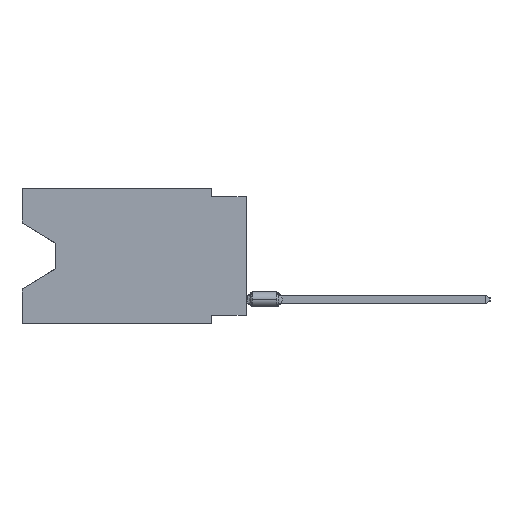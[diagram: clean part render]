
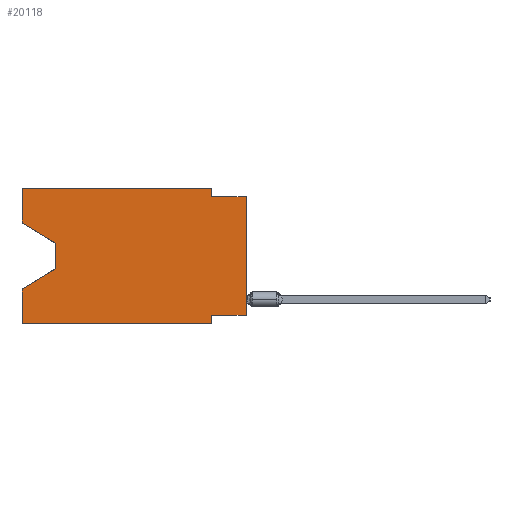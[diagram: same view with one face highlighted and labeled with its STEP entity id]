
A CAD part, left-side view. The second image highlights one B-rep face of the part: STEP entity #20118.
In plain terms, the highlighted planar face has unit normal (-1, 0, 0).
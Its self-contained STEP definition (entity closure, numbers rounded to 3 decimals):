
#1104 = VECTOR ( 'NONE', #51613, 1000. ) ;
#1359 = ORIENTED_EDGE ( 'NONE', *, *, #42672, .T. ) ;
#1464 = EDGE_CURVE ( 'NONE', #30477, #52670, #32960, .T. ) ;
#1602 = CARTESIAN_POINT ( 'NONE',  ( 0., 13.97, -5.893 ) ) ;
#2271 = EDGE_LOOP ( 'NONE', ( #1359, #35924, #19201, #23633, #43692, #17999, #37545, #6547, #33338, #36070, #18843, #28614 ) ) ;
#2519 = LINE ( 'NONE', #6891, #19369 ) ;
#3648 = DIRECTION ( 'NONE',  ( 0., 0., 1. ) ) ;
#3745 = DIRECTION ( 'NONE',  ( 0., 0., 1. ) ) ;
#4346 = FACE_OUTER_BOUND ( 'NONE', #2271, .T. ) ;
#5428 = LINE ( 'NONE', #1602, #26928 ) ;
#6082 = EDGE_CURVE ( 'NONE', #46566, #53628, #15417, .T. ) ;
#6547 = ORIENTED_EDGE ( 'NONE', *, *, #40196, .T. ) ;
#6814 = EDGE_CURVE ( 'NONE', #42949, #31738, #7811, .T. ) ;
#6891 = CARTESIAN_POINT ( 'NONE',  ( 0., 0., -0.635 ) ) ;
#7076 = DIRECTION ( 'NONE',  ( 0., 0., 1. ) ) ;
#7616 = LINE ( 'NONE', #41135, #11554 ) ;
#7811 = LINE ( 'NONE', #36995, #37672 ) ;
#8445 = CARTESIAN_POINT ( 'NONE',  ( 0., 0., -9.271 ) ) ;
#8460 = PLANE ( 'NONE',  #45434 ) ;
#8969 = VERTEX_POINT ( 'NONE', #32967 ) ;
#9122 = VERTEX_POINT ( 'NONE', #37843 ) ;
#10233 = EDGE_CURVE ( 'NONE', #49967, #9122, #53709, .T. ) ;
#11554 = VECTOR ( 'NONE', #7076, 1000. ) ;
#11574 = CARTESIAN_POINT ( 'NONE',  ( 0., 2.54, 0. ) ) ;
#12324 = CARTESIAN_POINT ( 'NONE',  ( 0., 2.54, -9.271 ) ) ;
#13862 = EDGE_CURVE ( 'NONE', #8969, #49967, #18412, .T. ) ;
#13881 = DIRECTION ( 'NONE',  ( 0., 0.855, -0.519 ) ) ;
#15417 = LINE ( 'NONE', #16221, #31559 ) ;
#15844 = VECTOR ( 'NONE', #34722, 1000. ) ;
#16221 = CARTESIAN_POINT ( 'NONE',  ( 0., 13.97, -4.013 ) ) ;
#17991 = CARTESIAN_POINT ( 'NONE',  ( 0., 13.97, -5.893 ) ) ;
#17999 = ORIENTED_EDGE ( 'NONE', *, *, #6814, .F. ) ;
#18412 = LINE ( 'NONE', #51601, #47965 ) ;
#18843 = ORIENTED_EDGE ( 'NONE', *, *, #13862, .F. ) ;
#19201 = ORIENTED_EDGE ( 'NONE', *, *, #26063, .T. ) ;
#19369 = VECTOR ( 'NONE', #32007, 1000. ) ;
#20118 = ADVANCED_FACE ( 'NONE', ( #4346 ), #8460, .F. ) ;
#21145 = CARTESIAN_POINT ( 'NONE',  ( 0., 0., 0. ) ) ;
#21344 = EDGE_CURVE ( 'NONE', #30477, #31738, #26867, .T. ) ;
#22269 = VECTOR ( 'NONE', #24584, 1000. ) ;
#22717 = CARTESIAN_POINT ( 'NONE',  ( 0., 16.383, -9.906 ) ) ;
#23620 = DIRECTION ( 'NONE',  ( 0., 0., -1. ) ) ;
#23633 = ORIENTED_EDGE ( 'NONE', *, *, #1464, .F. ) ;
#24114 = CARTESIAN_POINT ( 'NONE',  ( 0., 0., -0.635 ) ) ;
#24584 = DIRECTION ( 'NONE',  ( 0., 1., 0. ) ) ;
#24687 = EDGE_CURVE ( 'NONE', #51892, #42949, #53430, .T. ) ;
#24875 = DIRECTION ( 'NONE',  ( 0., 0., -1. ) ) ;
#25555 = CARTESIAN_POINT ( 'NONE',  ( 0., 0., -9.271 ) ) ;
#26021 = LINE ( 'NONE', #46432, #15844 ) ;
#26063 = EDGE_CURVE ( 'NONE', #53628, #52670, #5428, .T. ) ;
#26867 = LINE ( 'NONE', #30406, #1104 ) ;
#26928 = VECTOR ( 'NONE', #13881, 1000. ) ;
#28614 = ORIENTED_EDGE ( 'NONE', *, *, #47004, .F. ) ;
#29505 = CARTESIAN_POINT ( 'NONE',  ( 0., 16.383, -2.546 ) ) ;
#30016 = DIRECTION ( 'NONE',  ( 1., 0., 0. ) ) ;
#30406 = CARTESIAN_POINT ( 'NONE',  ( 0., 16.383, -9.906 ) ) ;
#30477 = VERTEX_POINT ( 'NONE', #22717 ) ;
#31559 = VECTOR ( 'NONE', #23620, 1000. ) ;
#31738 = VERTEX_POINT ( 'NONE', #38286 ) ;
#32007 = DIRECTION ( 'NONE',  ( 0., -1., 0. ) ) ;
#32960 = LINE ( 'NONE', #36052, #44784 ) ;
#32967 = CARTESIAN_POINT ( 'NONE',  ( 0., 16.383, 0. ) ) ;
#33338 = ORIENTED_EDGE ( 'NONE', *, *, #36591, .F. ) ;
#34722 = DIRECTION ( 'NONE',  ( 0., -0.855, -0.519 ) ) ;
#34854 = VERTEX_POINT ( 'NONE', #29505 ) ;
#35924 = ORIENTED_EDGE ( 'NONE', *, *, #6082, .T. ) ;
#36052 = CARTESIAN_POINT ( 'NONE',  ( 0., 16.383, 0. ) ) ;
#36070 = ORIENTED_EDGE ( 'NONE', *, *, #10233, .F. ) ;
#36591 = EDGE_CURVE ( 'NONE', #9122, #36642, #2519, .T. ) ;
#36642 = VERTEX_POINT ( 'NONE', #24114 ) ;
#36995 = CARTESIAN_POINT ( 'NONE',  ( 0., 2.54, -9.906 ) ) ;
#37545 = ORIENTED_EDGE ( 'NONE', *, *, #24687, .F. ) ;
#37672 = VECTOR ( 'NONE', #45429, 1000. ) ;
#37843 = CARTESIAN_POINT ( 'NONE',  ( 0., 2.54, -0.635 ) ) ;
#38286 = CARTESIAN_POINT ( 'NONE',  ( 0., 2.54, -9.906 ) ) ;
#38594 = CARTESIAN_POINT ( 'NONE',  ( 0., 13.97, -4.013 ) ) ;
#40196 = EDGE_CURVE ( 'NONE', #51892, #36642, #41805, .T. ) ;
#41135 = CARTESIAN_POINT ( 'NONE',  ( 0., 16.383, 0. ) ) ;
#41197 = CARTESIAN_POINT ( 'NONE',  ( 0., 2.54, 0. ) ) ;
#41440 = VECTOR ( 'NONE', #24875, 1000. ) ;
#41805 = LINE ( 'NONE', #21145, #47751 ) ;
#42672 = EDGE_CURVE ( 'NONE', #34854, #46566, #26021, .T. ) ;
#42949 = VERTEX_POINT ( 'NONE', #12324 ) ;
#43172 = DIRECTION ( 'NONE',  ( 0., -1., 0. ) ) ;
#43692 = ORIENTED_EDGE ( 'NONE', *, *, #21344, .T. ) ;
#44784 = VECTOR ( 'NONE', #3745, 1000. ) ;
#45429 = DIRECTION ( 'NONE',  ( 0., 0., -1. ) ) ;
#45434 = AXIS2_PLACEMENT_3D ( 'NONE', #50406, #30016, #46073 ) ;
#46073 = DIRECTION ( 'NONE',  ( 0., 0., -1. ) ) ;
#46432 = CARTESIAN_POINT ( 'NONE',  ( 0., 16.383, -2.546 ) ) ;
#46566 = VERTEX_POINT ( 'NONE', #38594 ) ;
#47004 = EDGE_CURVE ( 'NONE', #34854, #8969, #7616, .T. ) ;
#47751 = VECTOR ( 'NONE', #3648, 1000. ) ;
#47965 = VECTOR ( 'NONE', #43172, 1000. ) ;
#49967 = VERTEX_POINT ( 'NONE', #11574 ) ;
#50406 = CARTESIAN_POINT ( 'NONE',  ( 0., 16.383, 0. ) ) ;
#51601 = CARTESIAN_POINT ( 'NONE',  ( 0., 16.383, 0. ) ) ;
#51613 = DIRECTION ( 'NONE',  ( 0., -1., 0. ) ) ;
#51892 = VERTEX_POINT ( 'NONE', #25555 ) ;
#52670 = VERTEX_POINT ( 'NONE', #53223 ) ;
#53223 = CARTESIAN_POINT ( 'NONE',  ( 0., 16.383, -7.36 ) ) ;
#53430 = LINE ( 'NONE', #8445, #22269 ) ;
#53628 = VERTEX_POINT ( 'NONE', #17991 ) ;
#53709 = LINE ( 'NONE', #41197, #41440 ) ;
